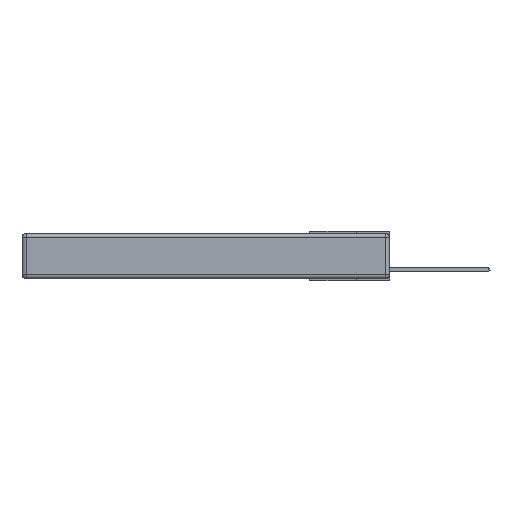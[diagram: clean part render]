
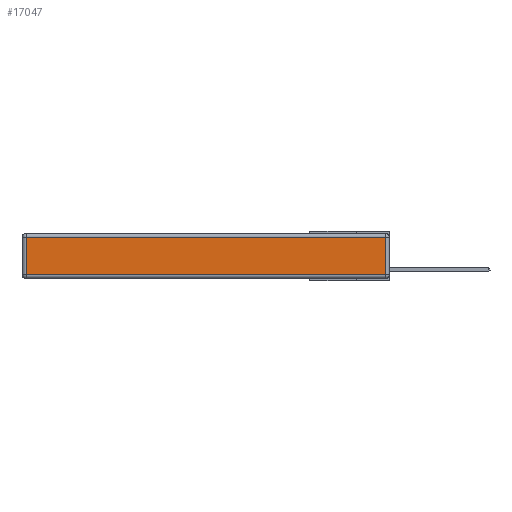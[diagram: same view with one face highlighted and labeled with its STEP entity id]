
A CAD part, left-side view. The second image highlights one B-rep face of the part: STEP entity #17047.
In plain terms, the highlighted planar face has unit normal (-1, 0, 0).
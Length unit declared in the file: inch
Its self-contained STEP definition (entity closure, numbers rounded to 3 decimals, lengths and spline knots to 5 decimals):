
#236 = LINE ( 'NONE', #29697, #6019 ) ;
#1225 = VERTEX_POINT ( 'NONE', #15819 ) ;
#2327 = VERTEX_POINT ( 'NONE', #8122 ) ;
#2504 = EDGE_LOOP ( 'NONE', ( #13292, #8523, #17346, #15797 ) ) ;
#2971 = VECTOR ( 'NONE', #24861, 39.37008 ) ;
#3226 = CARTESIAN_POINT ( 'NONE',  ( 0., 0., -0.313 ) ) ;
#3366 = EDGE_CURVE ( 'NONE', #31898, #2327, #236, .T. ) ;
#6019 = VECTOR ( 'NONE', #17667, 39.37008 ) ;
#6773 = CARTESIAN_POINT ( 'NONE',  ( 0., 0.03, -0.03 ) ) ;
#7346 = AXIS2_PLACEMENT_3D ( 'NONE', #21938, #22065, #29556 ) ;
#8122 = CARTESIAN_POINT ( 'NONE',  ( 0., 2.72, -0.313 ) ) ;
#8523 = ORIENTED_EDGE ( 'NONE', *, *, #29426, .T. ) ;
#11468 = VECTOR ( 'NONE', #13266, 39.37008 ) ;
#12263 = CARTESIAN_POINT ( 'NONE',  ( 0., 2.75, -0.03 ) ) ;
#13266 = DIRECTION ( 'NONE',  ( 0., -1., 0. ) ) ;
#13292 = ORIENTED_EDGE ( 'NONE', *, *, #29851, .T. ) ;
#13488 = FACE_OUTER_BOUND ( 'NONE', #2504, .T. ) ;
#15797 = ORIENTED_EDGE ( 'NONE', *, *, #3366, .T. ) ;
#15819 = CARTESIAN_POINT ( 'NONE',  ( 0., 0.03, -0.313 ) ) ;
#17047 = ADVANCED_FACE ( 'NONE', ( #13488 ), #21840, .T. ) ;
#17346 = ORIENTED_EDGE ( 'NONE', *, *, #17509, .T. ) ;
#17509 = EDGE_CURVE ( 'NONE', #28757, #31898, #28559, .T. ) ;
#17667 = DIRECTION ( 'NONE',  ( 0., 0., -1. ) ) ;
#19898 = CARTESIAN_POINT ( 'NONE',  ( 0., 0.03, -0.343 ) ) ;
#21840 = PLANE ( 'NONE',  #7346 ) ;
#21938 = CARTESIAN_POINT ( 'NONE',  ( 0., 0., -0.343 ) ) ;
#22065 = DIRECTION ( 'NONE',  ( -1., 0., 0. ) ) ;
#22083 = DIRECTION ( 'NONE',  ( 0., 1., 0. ) ) ;
#23404 = LINE ( 'NONE', #3226, #11468 ) ;
#24861 = DIRECTION ( 'NONE',  ( 0., 0., 1. ) ) ;
#25006 = LINE ( 'NONE', #19898, #2971 ) ;
#25516 = CARTESIAN_POINT ( 'NONE',  ( 0., 2.72, -0.03 ) ) ;
#27018 = VECTOR ( 'NONE', #22083, 39.37008 ) ;
#28559 = LINE ( 'NONE', #12263, #27018 ) ;
#28757 = VERTEX_POINT ( 'NONE', #6773 ) ;
#29426 = EDGE_CURVE ( 'NONE', #1225, #28757, #25006, .T. ) ;
#29556 = DIRECTION ( 'NONE',  ( 0., 0., 1. ) ) ;
#29697 = CARTESIAN_POINT ( 'NONE',  ( 0., 2.72, -0.343 ) ) ;
#29851 = EDGE_CURVE ( 'NONE', #2327, #1225, #23404, .T. ) ;
#31898 = VERTEX_POINT ( 'NONE', #25516 ) ;
